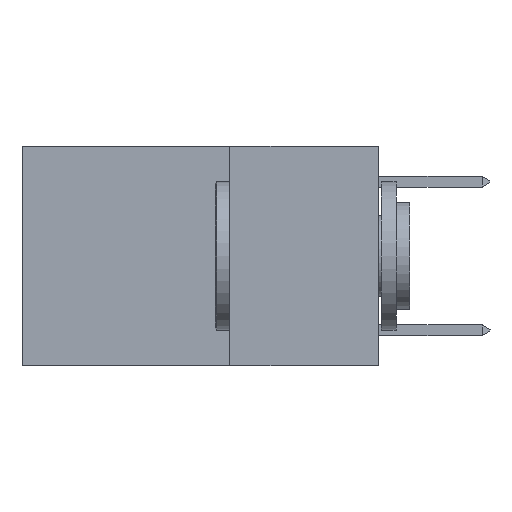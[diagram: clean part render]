
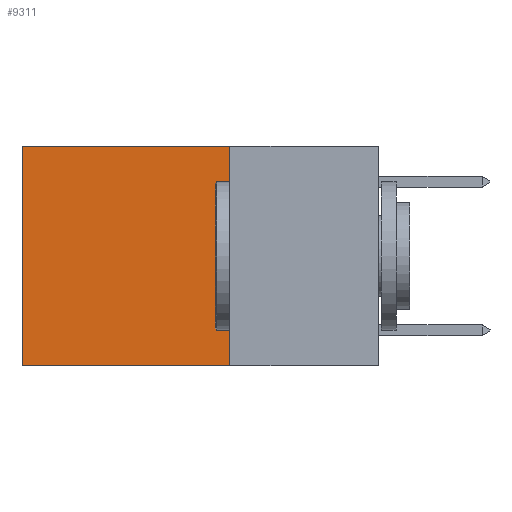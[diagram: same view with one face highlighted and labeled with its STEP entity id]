
A CAD part, left-side view. The second image highlights one B-rep face of the part: STEP entity #9311.
In plain terms, the highlighted planar face has unit normal (-1, 0, 0).
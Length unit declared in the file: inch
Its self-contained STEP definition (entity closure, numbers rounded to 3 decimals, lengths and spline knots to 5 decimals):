
#161 = VERTEX_POINT ( 'NONE', #3130 ) ;
#175 = CARTESIAN_POINT ( 'NONE',  ( 0.2625, 0.6, 0. ) ) ;
#298 = LINE ( 'NONE', #8606, #8594 ) ;
#1075 = ORIENTED_EDGE ( 'NONE', *, *, #9320, .T. ) ;
#1226 = CARTESIAN_POINT ( 'NONE',  ( 0.2625, 0.25, 0. ) ) ;
#1432 = LINE ( 'NONE', #1560, #2232 ) ;
#1560 = CARTESIAN_POINT ( 'NONE',  ( 0.2625, 0.25, 0. ) ) ;
#1668 = EDGE_CURVE ( 'NONE', #161, #3080, #8413, .T. ) ;
#1752 = ORIENTED_EDGE ( 'NONE', *, *, #9479, .T. ) ;
#1845 = VECTOR ( 'NONE', #4928, 39.37008 ) ;
#2232 = VECTOR ( 'NONE', #6574, 39.37008 ) ;
#2631 = VERTEX_POINT ( 'NONE', #4180 ) ;
#2970 = PLANE ( 'NONE',  #6577 ) ;
#3035 = DIRECTION ( 'NONE',  ( 0., 0., -1. ) ) ;
#3080 = VERTEX_POINT ( 'NONE', #9538 ) ;
#3130 = CARTESIAN_POINT ( 'NONE',  ( 0.2625, 0.25, 0. ) ) ;
#3884 = DIRECTION ( 'NONE',  ( 0., 0., -1. ) ) ;
#3964 = FACE_OUTER_BOUND ( 'NONE', #5602, .T. ) ;
#4180 = CARTESIAN_POINT ( 'NONE',  ( 0.2625, 0.6, 0. ) ) ;
#4312 = CARTESIAN_POINT ( 'NONE',  ( 0.2625, 0.6, -0.37 ) ) ;
#4928 = DIRECTION ( 'NONE',  ( 0., 0., -1. ) ) ;
#4993 = DIRECTION ( 'NONE',  ( 0., 1., 0. ) ) ;
#5340 = EDGE_CURVE ( 'NONE', #3080, #5701, #298, .T. ) ;
#5566 = ORIENTED_EDGE ( 'NONE', *, *, #5340, .F. ) ;
#5584 = LINE ( 'NONE', #175, #9496 ) ;
#5602 = EDGE_LOOP ( 'NONE', ( #1752, #5566, #5852, #1075 ) ) ;
#5701 = VERTEX_POINT ( 'NONE', #4312 ) ;
#5852 = ORIENTED_EDGE ( 'NONE', *, *, #1668, .F. ) ;
#6574 = DIRECTION ( 'NONE',  ( 0., 1., 0. ) ) ;
#6577 = AXIS2_PLACEMENT_3D ( 'NONE', #7392, #8196, #3035 ) ;
#7392 = CARTESIAN_POINT ( 'NONE',  ( 0.2625, 0.25, 0. ) ) ;
#8196 = DIRECTION ( 'NONE',  ( 1., 0., 0. ) ) ;
#8413 = LINE ( 'NONE', #1226, #1845 ) ;
#8594 = VECTOR ( 'NONE', #4993, 39.37008 ) ;
#8606 = CARTESIAN_POINT ( 'NONE',  ( 0.2625, 0.25, -0.37 ) ) ;
#9311 = ADVANCED_FACE ( 'NONE', ( #3964 ), #2970, .F. ) ;
#9320 = EDGE_CURVE ( 'NONE', #161, #2631, #1432, .T. ) ;
#9479 = EDGE_CURVE ( 'NONE', #2631, #5701, #5584, .T. ) ;
#9496 = VECTOR ( 'NONE', #3884, 39.37008 ) ;
#9538 = CARTESIAN_POINT ( 'NONE',  ( 0.2625, 0.25, -0.37 ) ) ;
